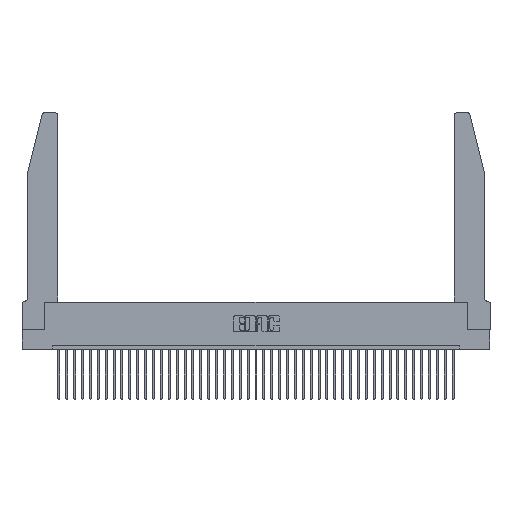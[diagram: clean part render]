
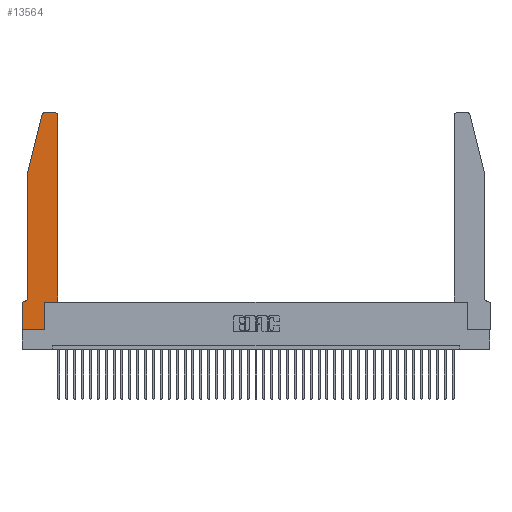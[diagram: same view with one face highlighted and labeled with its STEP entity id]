
A CAD part, top view. The second image highlights one B-rep face of the part: STEP entity #13564.
In plain terms, the highlighted planar face has unit normal (0, 0, 1).
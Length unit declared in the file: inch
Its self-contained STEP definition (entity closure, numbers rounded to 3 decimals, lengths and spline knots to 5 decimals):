
#183 = LINE ( 'NONE', #10615, #1727 ) ;
#674 = EDGE_CURVE ( 'NONE', #41794, #11532, #21182, .T. ) ;
#1727 = VECTOR ( 'NONE', #29747, 39.37008 ) ;
#2301 = DIRECTION ( 'NONE',  ( 0., 1., 0. ) ) ;
#2699 = LINE ( 'NONE', #4970, #3700 ) ;
#2867 = CARTESIAN_POINT ( 'NONE',  ( 0.0755, 2., 0.37 ) ) ;
#3080 = EDGE_CURVE ( 'NONE', #38586, #31758, #18523, .T. ) ;
#3700 = VECTOR ( 'NONE', #4553, 39.37008 ) ;
#4298 = LINE ( 'NONE', #28514, #14976 ) ;
#4457 = LINE ( 'NONE', #2867, #15604 ) ;
#4553 = DIRECTION ( 'NONE',  ( 1., 0., 0. ) ) ;
#4970 = CARTESIAN_POINT ( 'NONE',  ( 0., 0., 0.37 ) ) ;
#5724 = ORIENTED_EDGE ( 'NONE', *, *, #27497, .T. ) ;
#6075 = DIRECTION ( 'NONE',  ( 0., -1., 0. ) ) ;
#6083 = CARTESIAN_POINT ( 'NONE',  ( 0., 0.35, 0.37 ) ) ;
#6230 = CARTESIAN_POINT ( 'NONE',  ( 0.0755, 0.35, 0.37 ) ) ;
#6346 = DIRECTION ( 'NONE',  ( 0., 0., -1. ) ) ;
#6438 = LINE ( 'NONE', #31733, #6922 ) ;
#6922 = VECTOR ( 'NONE', #2301, 39.37008 ) ;
#8414 = VERTEX_POINT ( 'NONE', #32543 ) ;
#8665 = VERTEX_POINT ( 'NONE', #37525 ) ;
#8871 = CARTESIAN_POINT ( 'NONE',  ( 0.0755, 2., 0.37 ) ) ;
#9611 = DIRECTION ( 'NONE',  ( -1., 0., 0. ) ) ;
#9639 = CARTESIAN_POINT ( 'NONE',  ( 0., 0.35, 0.37 ) ) ;
#9881 = VECTOR ( 'NONE', #6075, 39.37008 ) ;
#9937 = VERTEX_POINT ( 'NONE', #18918 ) ;
#10615 = CARTESIAN_POINT ( 'NONE',  ( 0.2605, 2.75, 0.37 ) ) ;
#11188 = ORIENTED_EDGE ( 'NONE', *, *, #17661, .T. ) ;
#11391 = ORIENTED_EDGE ( 'NONE', *, *, #3080, .T. ) ;
#11506 = EDGE_CURVE ( 'NONE', #8665, #21694, #6438, .T. ) ;
#11532 = VERTEX_POINT ( 'NONE', #15039 ) ;
#11554 = AXIS2_PLACEMENT_3D ( 'NONE', #32057, #18867, #41660 ) ;
#11978 = CIRCLE ( 'NONE', #37314, 0.07 ) ;
#12411 = CARTESIAN_POINT ( 'NONE',  ( 0.4205, 2.75, 0.37 ) ) ;
#12919 = DIRECTION ( 'NONE',  ( 1., 0., 0. ) ) ;
#12971 = VERTEX_POINT ( 'NONE', #32405 ) ;
#13390 = FACE_OUTER_BOUND ( 'NONE', #24374, .T. ) ;
#13564 = ADVANCED_FACE ( 'NONE', ( #13390 ), #23230, .T. ) ;
#14976 = VECTOR ( 'NONE', #15770, 39.37008 ) ;
#15039 = CARTESIAN_POINT ( 'NONE',  ( 0.4505, 2.72, 0.37 ) ) ;
#15158 = AXIS2_PLACEMENT_3D ( 'NONE', #9639, #19419, #12919 ) ;
#15604 = VECTOR ( 'NONE', #38971, 39.37008 ) ;
#15770 = DIRECTION ( 'NONE',  ( 1., 0., 0. ) ) ;
#16409 = CARTESIAN_POINT ( 'NONE',  ( 0.0055, 0.42, 0.37 ) ) ;
#17162 = VECTOR ( 'NONE', #31841, 39.37008 ) ;
#17661 = EDGE_CURVE ( 'NONE', #11532, #28783, #37071, .T. ) ;
#17868 = DIRECTION ( 'NONE',  ( 0., 1., 0. ) ) ;
#18116 = CARTESIAN_POINT ( 'NONE',  ( 0.25487, 2.72718, 0.37 ) ) ;
#18516 = AXIS2_PLACEMENT_3D ( 'NONE', #35195, #38469, #19052 ) ;
#18523 = LINE ( 'NONE', #21849, #9881 ) ;
#18867 = DIRECTION ( 'NONE',  ( 0., 0., 1. ) ) ;
#18918 = CARTESIAN_POINT ( 'NONE',  ( 0.284, 2.75, 0.37 ) ) ;
#19052 = DIRECTION ( 'NONE',  ( 1., 0., 0. ) ) ;
#19148 = ORIENTED_EDGE ( 'NONE', *, *, #20067, .T. ) ;
#19419 = DIRECTION ( 'NONE',  ( 0., 0., 1. ) ) ;
#19586 = EDGE_CURVE ( 'NONE', #41490, #38586, #4457, .T. ) ;
#20067 = EDGE_CURVE ( 'NONE', #29496, #12971, #30329, .T. ) ;
#21182 = LINE ( 'NONE', #34566, #31303 ) ;
#21694 = VERTEX_POINT ( 'NONE', #28748 ) ;
#21849 = CARTESIAN_POINT ( 'NONE',  ( 0.0755, 2., 0.37 ) ) ;
#21946 = EDGE_CURVE ( 'NONE', #9937, #41490, #25425, .T. ) ;
#23063 = ORIENTED_EDGE ( 'NONE', *, *, #674, .T. ) ;
#23230 = PLANE ( 'NONE',  #15158 ) ;
#23784 = ORIENTED_EDGE ( 'NONE', *, *, #37501, .T. ) ;
#24374 = EDGE_LOOP ( 'NONE', ( #25858, #27776, #30745, #11391, #23784, #30699, #19148, #5724, #41322, #32950, #23063, #11188 ) ) ;
#25425 = CIRCLE ( 'NONE', #11554, 0.03 ) ;
#25858 = ORIENTED_EDGE ( 'NONE', *, *, #33366, .T. ) ;
#26033 = EDGE_CURVE ( 'NONE', #21694, #41794, #4298, .T. ) ;
#26649 = EDGE_CURVE ( 'NONE', #8414, #29496, #40227, .T. ) ;
#27497 = EDGE_CURVE ( 'NONE', #12971, #8665, #2699, .T. ) ;
#27776 = ORIENTED_EDGE ( 'NONE', *, *, #21946, .T. ) ;
#28070 = VECTOR ( 'NONE', #28772, 39.37008 ) ;
#28514 = CARTESIAN_POINT ( 'NONE',  ( 0.4505, 0.35, 0.37 ) ) ;
#28748 = CARTESIAN_POINT ( 'NONE',  ( 0.2865, 0.35, 0.37 ) ) ;
#28772 = DIRECTION ( 'NONE',  ( -1., 0., 0. ) ) ;
#28783 = VERTEX_POINT ( 'NONE', #12411 ) ;
#29496 = VERTEX_POINT ( 'NONE', #6083 ) ;
#29747 = DIRECTION ( 'NONE',  ( -1., 0., 0. ) ) ;
#30329 = LINE ( 'NONE', #32132, #17162 ) ;
#30699 = ORIENTED_EDGE ( 'NONE', *, *, #26649, .T. ) ;
#30729 = CARTESIAN_POINT ( 'NONE',  ( 0.0755, 0.42, 0.37 ) ) ;
#30745 = ORIENTED_EDGE ( 'NONE', *, *, #19586, .T. ) ;
#31303 = VECTOR ( 'NONE', #17868, 39.37008 ) ;
#31733 = CARTESIAN_POINT ( 'NONE',  ( 0.2865, 0.35, 0.37 ) ) ;
#31758 = VERTEX_POINT ( 'NONE', #30729 ) ;
#31841 = DIRECTION ( 'NONE',  ( 0., -1., 0. ) ) ;
#32057 = CARTESIAN_POINT ( 'NONE',  ( 0.284, 2.72, 0.37 ) ) ;
#32132 = CARTESIAN_POINT ( 'NONE',  ( 0., 0., 0.37 ) ) ;
#32405 = CARTESIAN_POINT ( 'NONE',  ( 0., 0., 0.37 ) ) ;
#32543 = CARTESIAN_POINT ( 'NONE',  ( 0.0055, 0.35, 0.37 ) ) ;
#32950 = ORIENTED_EDGE ( 'NONE', *, *, #26033, .T. ) ;
#33366 = EDGE_CURVE ( 'NONE', #28783, #9937, #183, .T. ) ;
#34566 = CARTESIAN_POINT ( 'NONE',  ( 0.4505, 0.35, 0.37 ) ) ;
#35195 = CARTESIAN_POINT ( 'NONE',  ( 0.4205, 2.72, 0.37 ) ) ;
#36571 = CARTESIAN_POINT ( 'NONE',  ( 0.4505, 0.35, 0.37 ) ) ;
#37071 = CIRCLE ( 'NONE', #18516, 0.03 ) ;
#37314 = AXIS2_PLACEMENT_3D ( 'NONE', #16409, #6346, #9611 ) ;
#37501 = EDGE_CURVE ( 'NONE', #31758, #8414, #11978, .T. ) ;
#37525 = CARTESIAN_POINT ( 'NONE',  ( 0.2865, 0., 0.37 ) ) ;
#38469 = DIRECTION ( 'NONE',  ( 0., 0., 1. ) ) ;
#38586 = VERTEX_POINT ( 'NONE', #8871 ) ;
#38971 = DIRECTION ( 'NONE',  ( -0.239, -0.971, 0. ) ) ;
#40227 = LINE ( 'NONE', #6230, #28070 ) ;
#41322 = ORIENTED_EDGE ( 'NONE', *, *, #11506, .T. ) ;
#41490 = VERTEX_POINT ( 'NONE', #18116 ) ;
#41660 = DIRECTION ( 'NONE',  ( 1., 0., 0. ) ) ;
#41794 = VERTEX_POINT ( 'NONE', #36571 ) ;
